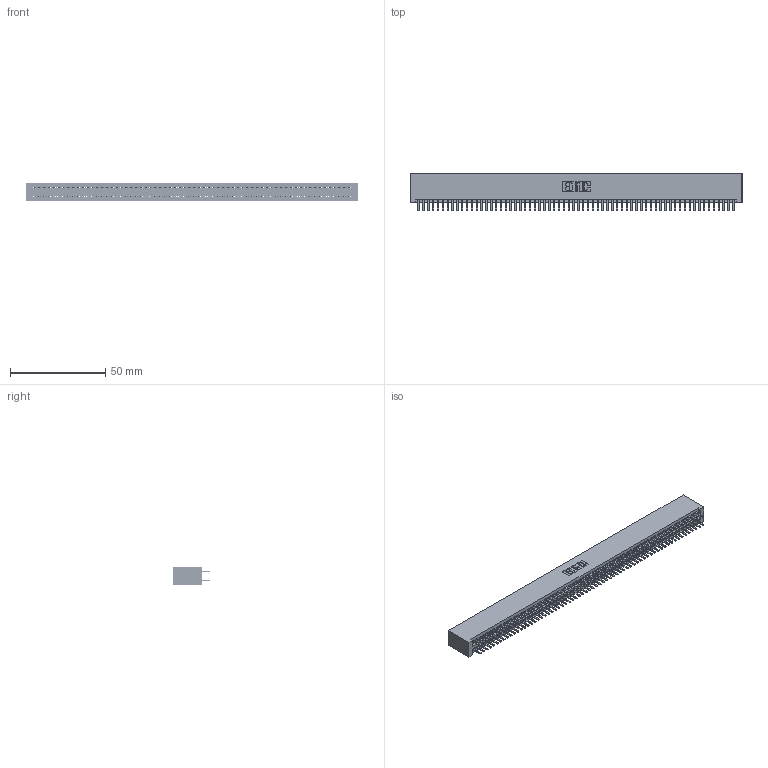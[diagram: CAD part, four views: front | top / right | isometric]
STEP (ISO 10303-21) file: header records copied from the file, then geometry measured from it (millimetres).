
FILE_DESCRIPTION (( 'STEP AP203' ), '1' );
FILE_NAME ('345-132-520-201.STEP', '2018-10-20T03:09:05', ( '' ), ( '' ), 'SwSTEP 2.0', 'SolidWorks 2016', '' );
FILE_SCHEMA (( 'CONFIG_CONTROL_DESIGN' ));
Length unit declared in the file: inch
Products named in the file (3): 345-132-520-201; 345 Part_No Mounting Lugs; 345-292-001_345-293-120
Assembly tree (133 placements, depth 2):
  345-132-520-201
    345 Part_No Mounting Lugs
    345-292-001_345-293-120  x132
Bounding box: 174.24 x 19.68 x 9.4 mm (x, y, z)
Volume: 17706.9 mm3; surface area: 26818.4 mm2
Topology: 133 solids, 133 shells, 7246 faces, 21041 edges, 13674 vertices
Faces by surface type: plane 4696, cylinder 2550
Entity records: 48391 total; most frequent: CARTESIAN_POINT 8100, ORIENTED_EDGE 8022, DIRECTION 7095, EDGE_CURVE 4011, LINE 3619, VECTOR 3619, VERTEX_POINT 2670, AXIS2_PLACEMENT_3D 1738
